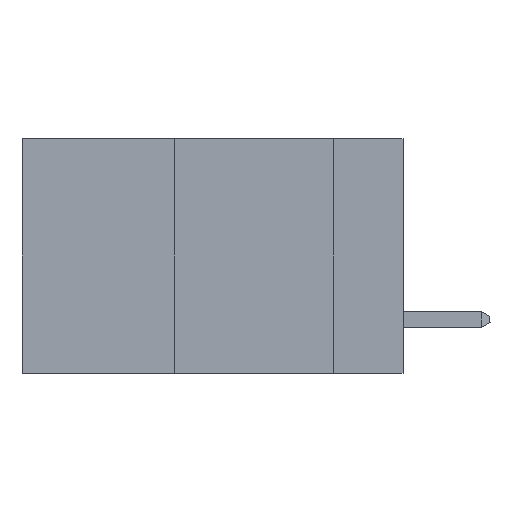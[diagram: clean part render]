
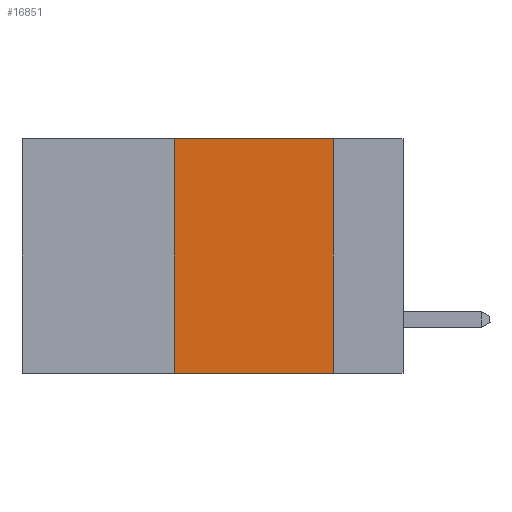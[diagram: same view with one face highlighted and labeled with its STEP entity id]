
A CAD part, left-side view. The second image highlights one B-rep face of the part: STEP entity #16851.
In plain terms, the highlighted planar face has unit normal (-1, 0, 0).
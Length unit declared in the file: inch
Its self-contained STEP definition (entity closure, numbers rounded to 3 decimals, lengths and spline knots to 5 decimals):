
#1204 = VECTOR ( 'NONE', #2327, 39.37008 ) ;
#1248 = VECTOR ( 'NONE', #5277, 39.37008 ) ;
#1316 = LINE ( 'NONE', #15840, #14174 ) ;
#1430 = LINE ( 'NONE', #12812, #15361 ) ;
#2327 = DIRECTION ( 'NONE',  ( 0., 0., -1. ) ) ;
#3362 = VERTEX_POINT ( 'NONE', #4838 ) ;
#4463 = VERTEX_POINT ( 'NONE', #6289 ) ;
#4788 = ORIENTED_EDGE ( 'NONE', *, *, #13516, .F. ) ;
#4838 = CARTESIAN_POINT ( 'NONE',  ( 0., 0.11, -0.37 ) ) ;
#5277 = DIRECTION ( 'NONE',  ( 0., -1., 0. ) ) ;
#6077 = VERTEX_POINT ( 'NONE', #6809 ) ;
#6289 = CARTESIAN_POINT ( 'NONE',  ( 0., 0.36, -0.37 ) ) ;
#6809 = CARTESIAN_POINT ( 'NONE',  ( 0., 0.36, 0. ) ) ;
#7099 = EDGE_CURVE ( 'NONE', #6077, #12487, #11339, .T. ) ;
#7831 = CARTESIAN_POINT ( 'NONE',  ( 0., 0.6, 0. ) ) ;
#9264 = CARTESIAN_POINT ( 'NONE',  ( 0., 0.11, 0. ) ) ;
#10053 = AXIS2_PLACEMENT_3D ( 'NONE', #7831, #13198, #15843 ) ;
#10340 = EDGE_CURVE ( 'NONE', #4463, #3362, #1430, .T. ) ;
#10456 = DIRECTION ( 'NONE',  ( 0., 0., 1. ) ) ;
#10584 = ORIENTED_EDGE ( 'NONE', *, *, #7099, .F. ) ;
#11049 = EDGE_CURVE ( 'NONE', #12487, #3362, #12140, .T. ) ;
#11339 = LINE ( 'NONE', #14478, #1248 ) ;
#11454 = FACE_OUTER_BOUND ( 'NONE', #12733, .T. ) ;
#12140 = LINE ( 'NONE', #12919, #1204 ) ;
#12487 = VERTEX_POINT ( 'NONE', #9264 ) ;
#12733 = EDGE_LOOP ( 'NONE', ( #13212, #10584, #4788, #14082 ) ) ;
#12812 = CARTESIAN_POINT ( 'NONE',  ( 0., 0.6, -0.37 ) ) ;
#12919 = CARTESIAN_POINT ( 'NONE',  ( 0., 0.11, 0. ) ) ;
#13198 = DIRECTION ( 'NONE',  ( 1., 0., 0. ) ) ;
#13212 = ORIENTED_EDGE ( 'NONE', *, *, #11049, .F. ) ;
#13516 = EDGE_CURVE ( 'NONE', #4463, #6077, #1316, .T. ) ;
#14082 = ORIENTED_EDGE ( 'NONE', *, *, #10340, .T. ) ;
#14174 = VECTOR ( 'NONE', #10456, 39.37008 ) ;
#14478 = CARTESIAN_POINT ( 'NONE',  ( 0., 0.6, 0. ) ) ;
#14637 = PLANE ( 'NONE',  #10053 ) ;
#15361 = VECTOR ( 'NONE', #15586, 39.37008 ) ;
#15586 = DIRECTION ( 'NONE',  ( 0., -1., 0. ) ) ;
#15840 = CARTESIAN_POINT ( 'NONE',  ( 0., 0.36, 0. ) ) ;
#15843 = DIRECTION ( 'NONE',  ( 0., 0., -1. ) ) ;
#16851 = ADVANCED_FACE ( 'NONE', ( #11454 ), #14637, .F. ) ;
